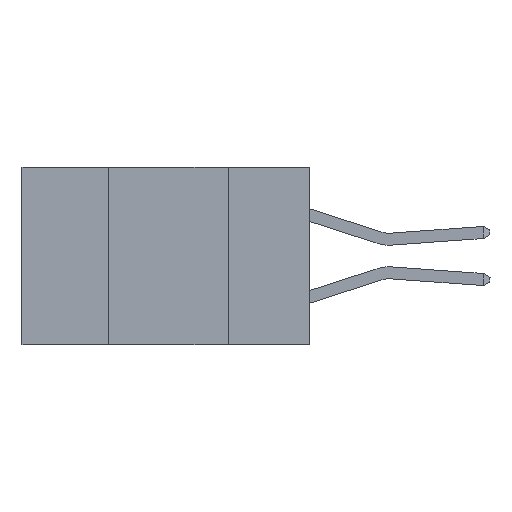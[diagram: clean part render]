
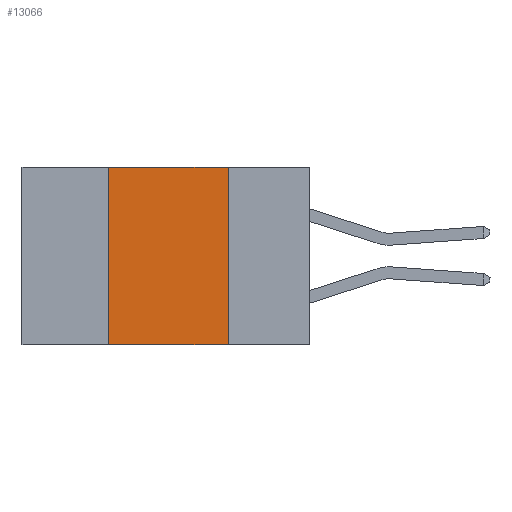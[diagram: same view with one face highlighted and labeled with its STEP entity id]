
A CAD part, left-side view. The second image highlights one B-rep face of the part: STEP entity #13066.
In plain terms, the highlighted planar face has unit normal (-1, 0, 0).
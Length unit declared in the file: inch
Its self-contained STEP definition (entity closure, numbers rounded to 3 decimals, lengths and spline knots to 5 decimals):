
#242 = CARTESIAN_POINT ( 'NONE',  ( 0., 0.42, 0. ) ) ;
#383 = LINE ( 'NONE', #9120, #15318 ) ;
#541 = DIRECTION ( 'NONE',  ( 0., 0., -1. ) ) ;
#1104 = VECTOR ( 'NONE', #541, 39.37008 ) ;
#1313 = CARTESIAN_POINT ( 'NONE',  ( 0., 0.42, -0.37 ) ) ;
#2818 = ORIENTED_EDGE ( 'NONE', *, *, #13945, .F. ) ;
#3885 = EDGE_LOOP ( 'NONE', ( #17153, #2818, #5814, #7471 ) ) ;
#4321 = VERTEX_POINT ( 'NONE', #242 ) ;
#4628 = AXIS2_PLACEMENT_3D ( 'NONE', #13195, #4705, #14651 ) ;
#4705 = DIRECTION ( 'NONE',  ( 1., 0., 0. ) ) ;
#4881 = VECTOR ( 'NONE', #5873, 39.37008 ) ;
#5814 = ORIENTED_EDGE ( 'NONE', *, *, #11170, .F. ) ;
#5873 = DIRECTION ( 'NONE',  ( 0., -1., 0. ) ) ;
#6062 = PLANE ( 'NONE',  #4628 ) ;
#7302 = DIRECTION ( 'NONE',  ( 0., 0., 1. ) ) ;
#7471 = ORIENTED_EDGE ( 'NONE', *, *, #10217, .T. ) ;
#9120 = CARTESIAN_POINT ( 'NONE',  ( 0., 0.6, -0.37 ) ) ;
#9823 = LINE ( 'NONE', #14934, #1104 ) ;
#10217 = EDGE_CURVE ( 'NONE', #18240, #12137, #383, .T. ) ;
#10466 = VECTOR ( 'NONE', #7302, 39.37008 ) ;
#10523 = DIRECTION ( 'NONE',  ( 0., -1., 0. ) ) ;
#11052 = FACE_OUTER_BOUND ( 'NONE', #3885, .T. ) ;
#11170 = EDGE_CURVE ( 'NONE', #18240, #4321, #14158, .T. ) ;
#12137 = VERTEX_POINT ( 'NONE', #18392 ) ;
#12433 = LINE ( 'NONE', #18657, #4881 ) ;
#13066 = ADVANCED_FACE ( 'NONE', ( #11052 ), #6062, .F. ) ;
#13195 = CARTESIAN_POINT ( 'NONE',  ( 0., 0.6, 0. ) ) ;
#13945 = EDGE_CURVE ( 'NONE', #4321, #15641, #12433, .T. ) ;
#14158 = LINE ( 'NONE', #1313, #10466 ) ;
#14651 = DIRECTION ( 'NONE',  ( 0., 0., -1. ) ) ;
#14912 = EDGE_CURVE ( 'NONE', #15641, #12137, #9823, .T. ) ;
#14934 = CARTESIAN_POINT ( 'NONE',  ( 0., 0.17, -0.37 ) ) ;
#15318 = VECTOR ( 'NONE', #10523, 39.37008 ) ;
#15641 = VERTEX_POINT ( 'NONE', #17810 ) ;
#17153 = ORIENTED_EDGE ( 'NONE', *, *, #14912, .F. ) ;
#17620 = CARTESIAN_POINT ( 'NONE',  ( 0., 0.42, -0.37 ) ) ;
#17810 = CARTESIAN_POINT ( 'NONE',  ( 0., 0.17, 0. ) ) ;
#18240 = VERTEX_POINT ( 'NONE', #17620 ) ;
#18392 = CARTESIAN_POINT ( 'NONE',  ( 0., 0.17, -0.37 ) ) ;
#18657 = CARTESIAN_POINT ( 'NONE',  ( 0., 0.6, 0. ) ) ;
